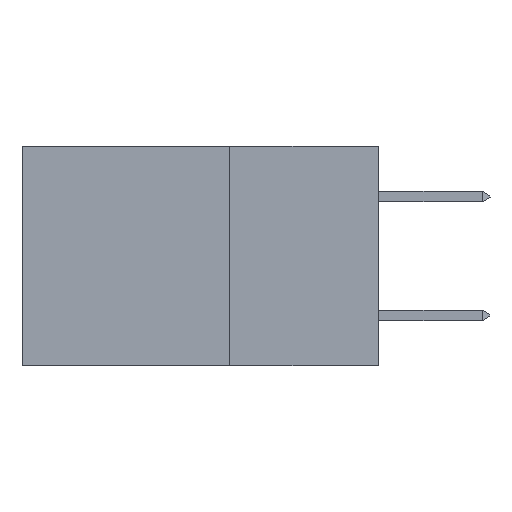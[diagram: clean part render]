
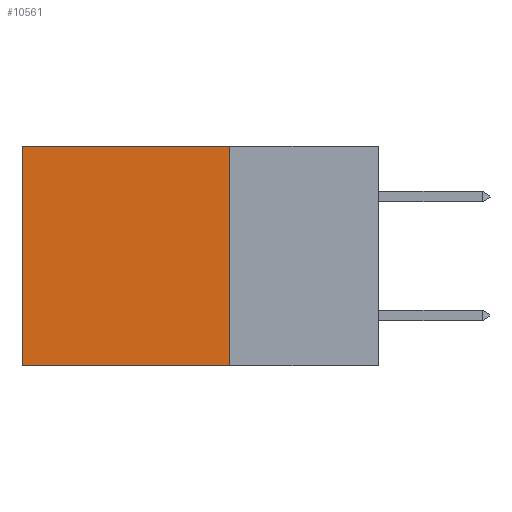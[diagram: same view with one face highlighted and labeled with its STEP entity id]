
A CAD part, left-side view. The second image highlights one B-rep face of the part: STEP entity #10561.
In plain terms, the highlighted planar face has unit normal (-1, 0, 0).
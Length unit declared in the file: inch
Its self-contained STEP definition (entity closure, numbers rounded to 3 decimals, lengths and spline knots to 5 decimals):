
#971 = CARTESIAN_POINT ( 'NONE',  ( 0.298, 0.6, 0. ) ) ;
#1740 = VECTOR ( 'NONE', #3942, 39.37008 ) ;
#2482 = VERTEX_POINT ( 'NONE', #12639 ) ;
#2895 = FACE_OUTER_BOUND ( 'NONE', #11139, .T. ) ;
#2984 = CARTESIAN_POINT ( 'NONE',  ( 0.298, 0.25, 0. ) ) ;
#3942 = DIRECTION ( 'NONE',  ( 0., 1., 0. ) ) ;
#4609 = EDGE_CURVE ( 'NONE', #2482, #7430, #20421, .T. ) ;
#5042 = VECTOR ( 'NONE', #18551, 39.37008 ) ;
#5568 = AXIS2_PLACEMENT_3D ( 'NONE', #2984, #8026, #19211 ) ;
#5589 = VECTOR ( 'NONE', #14200, 39.37008 ) ;
#6394 = PLANE ( 'NONE',  #5568 ) ;
#7430 = VERTEX_POINT ( 'NONE', #15570 ) ;
#7726 = VECTOR ( 'NONE', #9282, 39.37008 ) ;
#8026 = DIRECTION ( 'NONE',  ( 1., 0., 0. ) ) ;
#8111 = ORIENTED_EDGE ( 'NONE', *, *, #20602, .T. ) ;
#8402 = ORIENTED_EDGE ( 'NONE', *, *, #10281, .F. ) ;
#8996 = CARTESIAN_POINT ( 'NONE',  ( 0.298, 0.25, 0. ) ) ;
#9057 = CARTESIAN_POINT ( 'NONE',  ( 0.298, 0.25, 0. ) ) ;
#9199 = CARTESIAN_POINT ( 'NONE',  ( 0.298, 0.25, -0.37 ) ) ;
#9282 = DIRECTION ( 'NONE',  ( 0., 1., 0. ) ) ;
#9489 = LINE ( 'NONE', #8996, #5042 ) ;
#10134 = LINE ( 'NONE', #15387, #1740 ) ;
#10188 = ORIENTED_EDGE ( 'NONE', *, *, #4609, .T. ) ;
#10281 = EDGE_CURVE ( 'NONE', #12545, #15517, #10134, .T. ) ;
#10561 = ADVANCED_FACE ( 'NONE', ( #2895 ), #6394, .F. ) ;
#11139 = EDGE_LOOP ( 'NONE', ( #8111, #8402, #19757, #10188 ) ) ;
#12545 = VERTEX_POINT ( 'NONE', #9199 ) ;
#12639 = CARTESIAN_POINT ( 'NONE',  ( 0.298, 0.25, 0. ) ) ;
#14200 = DIRECTION ( 'NONE',  ( 0., 0., -1. ) ) ;
#15387 = CARTESIAN_POINT ( 'NONE',  ( 0.298, 0.25, -0.37 ) ) ;
#15517 = VERTEX_POINT ( 'NONE', #18828 ) ;
#15570 = CARTESIAN_POINT ( 'NONE',  ( 0.298, 0.6, 0. ) ) ;
#16004 = EDGE_CURVE ( 'NONE', #2482, #12545, #9489, .T. ) ;
#18551 = DIRECTION ( 'NONE',  ( 0., 0., -1. ) ) ;
#18828 = CARTESIAN_POINT ( 'NONE',  ( 0.298, 0.6, -0.37 ) ) ;
#18937 = LINE ( 'NONE', #971, #5589 ) ;
#19211 = DIRECTION ( 'NONE',  ( 0., 0., -1. ) ) ;
#19757 = ORIENTED_EDGE ( 'NONE', *, *, #16004, .F. ) ;
#20421 = LINE ( 'NONE', #9057, #7726 ) ;
#20602 = EDGE_CURVE ( 'NONE', #7430, #15517, #18937, .T. ) ;
